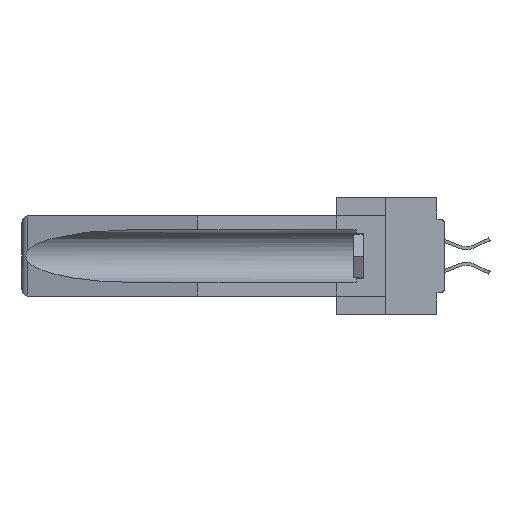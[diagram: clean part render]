
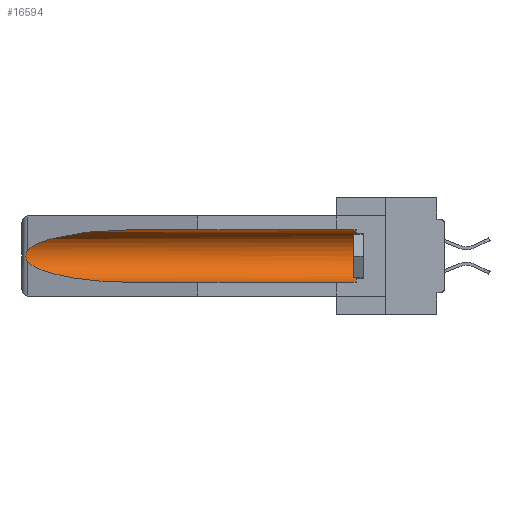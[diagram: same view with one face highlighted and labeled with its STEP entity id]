
A CAD part, left-side view. The second image highlights one B-rep face of the part: STEP entity #16594.
In plain terms, the highlighted cylindrical face has radius 2.857 mm (diameter 5.715 mm), a partial arc.
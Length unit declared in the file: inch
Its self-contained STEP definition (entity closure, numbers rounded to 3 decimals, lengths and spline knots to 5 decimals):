
#472 = ORIENTED_EDGE ( 'NONE', *, *, #34705, .T. ) ;
#797 = VERTEX_POINT ( 'NONE', #30184 ) ;
#2917 = CIRCLE ( 'NONE', #24314, 0.1125 ) ;
#3531 = ORIENTED_EDGE ( 'NONE', *, *, #27631, .T. ) ;
#4348 = VECTOR ( 'NONE', #25185, 39.37008 ) ;
#4853 = ORIENTED_EDGE ( 'NONE', *, *, #28065, .T. ) ;
#5265 = ORIENTED_EDGE ( 'NONE', *, *, #26922, .F. ) ;
#5546 = CARTESIAN_POINT ( 'NONE',  ( 0.25451, 1.48313, -0.09465 ) ) ;
#5923 = CARTESIAN_POINT ( 'NONE',  ( 0.155, -0.30754, -0.059 ) ) ;
#6290 = DIRECTION ( 'NONE',  ( 0., 1., 0. ) ) ;
#7435 = CARTESIAN_POINT ( 'NONE',  ( 0.2673, 1.53269, -0.17917 ) ) ;
#7820 = CARTESIAN_POINT ( 'NONE',  ( 0.2675, 1.53308, -0.16763 ) ) ;
#7835 = CARTESIAN_POINT ( 'NONE',  ( 0.155, -0.30754, -0.284 ) ) ;
#7995 = CARTESIAN_POINT ( 'NONE',  ( 0.155, 0.126, -0.284 ) ) ;
#8628 = VERTEX_POINT ( 'NONE', #7995 ) ;
#9781 = DIRECTION ( 'NONE',  ( 0., -1., 0. ) ) ;
#10175 = CARTESIAN_POINT ( 'NONE',  ( 0.26597, 1.52961, -0.15275 ) ) ;
#10273 = CARTESIAN_POINT ( 'NONE',  ( 0.155, 1.07973, -0.284 ) ) ;
#10451 = VERTEX_POINT ( 'NONE', #35290 ) ;
#10676 = CARTESIAN_POINT ( 'NONE',  ( 0.2673, 1.5327, -0.16383 ) ) ;
#11134 = AXIS2_PLACEMENT_3D ( 'NONE', #32999, #6290, #27169 ) ;
#11292 = LINE ( 'NONE', #7835, #4348 ) ;
#11300 = CYLINDRICAL_SURFACE ( 'NONE', #11134, 0.1125 ) ;
#14345 = DIRECTION ( 'NONE',  ( 0., 1., 0. ) ) ;
#14862 = LINE ( 'NONE', #5923, #37716 ) ;
#15504 =( BOUNDED_CURVE ( )  B_SPLINE_CURVE ( 3, ( #17402, #38463, #5546, #29418 ),
 .UNSPECIFIED., .F., .F. ) 
 B_SPLINE_CURVE_WITH_KNOTS ( ( 4, 4 ),
 ( 4.71239, 6.08839 ),
 .UNSPECIFIED. ) 
 CURVE ( )  GEOMETRIC_REPRESENTATION_ITEM ( )  RATIONAL_B_SPLINE_CURVE ( ( 1., 0.848, 0.848, 1. ) ) 
 REPRESENTATION_ITEM ( '' )  );
#16244 =( BOUNDED_CURVE ( )  B_SPLINE_CURVE ( 3, ( #27955, #22053, #30961, #33921 ),
 .UNSPECIFIED., .F., .F. ) 
 B_SPLINE_CURVE_WITH_KNOTS ( ( 4, 4 ),
 ( 0.1948, 1.5708 ),
 .UNSPECIFIED. ) 
 CURVE ( )  GEOMETRIC_REPRESENTATION_ITEM ( )  RATIONAL_B_SPLINE_CURVE ( ( 1., 0.848, 0.848, 1. ) ) 
 REPRESENTATION_ITEM ( '' )  );
#16594 = ADVANCED_FACE ( 'NONE', ( #28157 ), #11300, .F. ) ;
#17397 = EDGE_CURVE ( 'NONE', #27054, #797, #15504, .T. ) ;
#17402 = CARTESIAN_POINT ( 'NONE',  ( 0.155, 1.07973, -0.059 ) ) ;
#17929 = EDGE_LOOP ( 'NONE', ( #29605, #4853, #30758, #5265, #472, #3531 ) ) ;
#19052 = CARTESIAN_POINT ( 'NONE',  ( 0.155, 0.126, -0.1715 ) ) ;
#21253 = B_SPLINE_CURVE_WITH_KNOTS ( 'NONE', 3,
 ( #36514, #10175, #28569, #10676, #7820, #31198, #7435, #37024, #28320, #28705 ),
 .UNSPECIFIED., .F., .F.,
 ( 4, 2, 2, 2, 4 ),
 ( 0., 0.00029, 0.00058, 0.00087, 0.00117 ),
 .UNSPECIFIED. ) ;
#22053 = CARTESIAN_POINT ( 'NONE',  ( 0.25451, 1.48313, -0.24835 ) ) ;
#22844 = CARTESIAN_POINT ( 'NONE',  ( 0.155, 1.07973, -0.059 ) ) ;
#24314 = AXIS2_PLACEMENT_3D ( 'NONE', #19052, #9781, #36389 ) ;
#25185 = DIRECTION ( 'NONE',  ( 0., 1., 0. ) ) ;
#26098 = EDGE_CURVE ( 'NONE', #28646, #31023, #16244, .T. ) ;
#26922 = EDGE_CURVE ( 'NONE', #8628, #31023, #11292, .T. ) ;
#27054 = VERTEX_POINT ( 'NONE', #22844 ) ;
#27169 = DIRECTION ( 'NONE',  ( 0., 0., 1. ) ) ;
#27631 = EDGE_CURVE ( 'NONE', #10451, #27054, #14862, .T. ) ;
#27955 = CARTESIAN_POINT ( 'NONE',  ( 0.26537, 1.52718, -0.19328 ) ) ;
#28065 = EDGE_CURVE ( 'NONE', #797, #28646, #21253, .T. ) ;
#28157 = FACE_OUTER_BOUND ( 'NONE', #17929, .T. ) ;
#28320 = CARTESIAN_POINT ( 'NONE',  ( 0.26597, 1.5296, -0.19026 ) ) ;
#28569 = CARTESIAN_POINT ( 'NONE',  ( 0.26654, 1.53092, -0.15636 ) ) ;
#28646 = VERTEX_POINT ( 'NONE', #31157 ) ;
#28705 = CARTESIAN_POINT ( 'NONE',  ( 0.26537, 1.52718, -0.19328 ) ) ;
#29418 = CARTESIAN_POINT ( 'NONE',  ( 0.26537, 1.52718, -0.14972 ) ) ;
#29605 = ORIENTED_EDGE ( 'NONE', *, *, #17397, .T. ) ;
#30184 = CARTESIAN_POINT ( 'NONE',  ( 0.26537, 1.52718, -0.14972 ) ) ;
#30758 = ORIENTED_EDGE ( 'NONE', *, *, #26098, .T. ) ;
#30961 = CARTESIAN_POINT ( 'NONE',  ( 0.21114, 1.30732, -0.284 ) ) ;
#31023 = VERTEX_POINT ( 'NONE', #10273 ) ;
#31157 = CARTESIAN_POINT ( 'NONE',  ( 0.26537, 1.52718, -0.19328 ) ) ;
#31198 = CARTESIAN_POINT ( 'NONE',  ( 0.2675, 1.53308, -0.17534 ) ) ;
#32999 = CARTESIAN_POINT ( 'NONE',  ( 0.155, -0.30754, -0.1715 ) ) ;
#33921 = CARTESIAN_POINT ( 'NONE',  ( 0.155, 1.07973, -0.284 ) ) ;
#34705 = EDGE_CURVE ( 'NONE', #8628, #10451, #2917, .T. ) ;
#35290 = CARTESIAN_POINT ( 'NONE',  ( 0.155, 0.126, -0.059 ) ) ;
#36389 = DIRECTION ( 'NONE',  ( 0., 0., 1. ) ) ;
#36514 = CARTESIAN_POINT ( 'NONE',  ( 0.26537, 1.52718, -0.14972 ) ) ;
#37024 = CARTESIAN_POINT ( 'NONE',  ( 0.26655, 1.53094, -0.18657 ) ) ;
#37716 = VECTOR ( 'NONE', #14345, 39.37008 ) ;
#38463 = CARTESIAN_POINT ( 'NONE',  ( 0.21114, 1.30732, -0.059 ) ) ;
